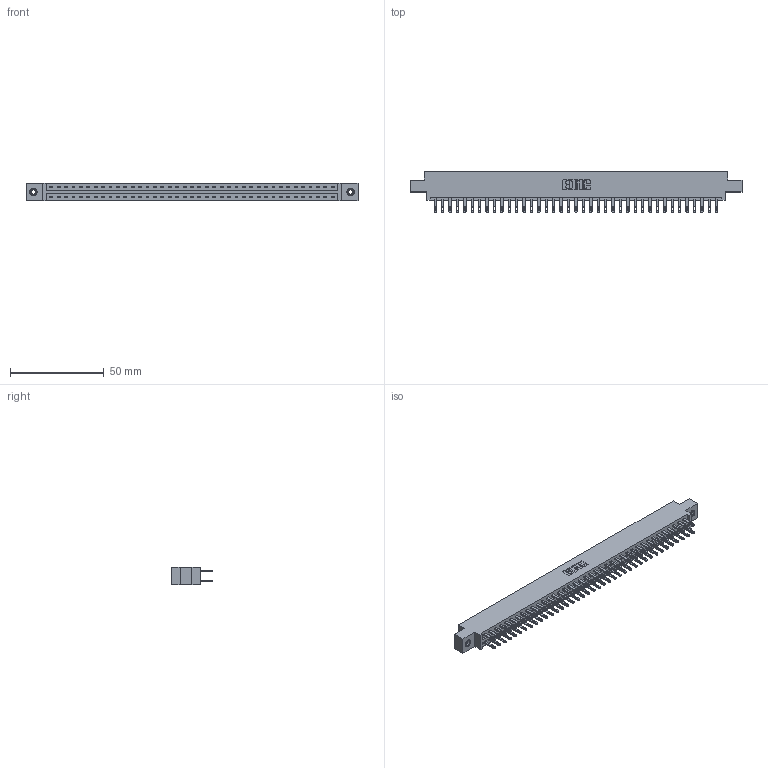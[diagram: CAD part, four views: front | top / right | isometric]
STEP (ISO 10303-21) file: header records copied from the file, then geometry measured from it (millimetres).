
FILE_DESCRIPTION (( 'STEP AP203' ), '1' );
FILE_NAME ('887-078-500-808.STEP', '2020-09-21T04:14:15', ( '' ), ( '' ), 'SwSTEP 2.0', 'SolidWorks 2020', '' );
FILE_SCHEMA (( 'CONFIG_CONTROL_DESIGN' ));
Length unit declared in the file: inch
Products named in the file (4): 345-292-001_345-293-100; 837 Part_0.170 Offset - 0.156 Dia-TI; 887-078-500-808; 345-250-001_345-250-003-102
Assembly tree (81 placements, depth 2):
  887-078-500-808
    837 Part_0.170 Offset - 0.156 Dia-TI
    345-292-001_345-293-100  x78
    345-250-001_345-250-003-102  x2
Bounding box: 177.55 x 21.85 x 9.4 mm (x, y, z)
Volume: 18785.6 mm3; surface area: 22205.3 mm2
Topology: 81 solids, 81 shells, 4078 faces, 12393 edges, 8254 vertices
Faces by surface type: plane 2602, cylinder 1460, cone 12, torus 4
Entity records: 31874 total; most frequent: CARTESIAN_POINT 5353, ORIENTED_EDGE 5282, DIRECTION 4591, EDGE_CURVE 2641, LINE 2489, VECTOR 2489, VERTEX_POINT 1756, AXIS2_PLACEMENT_3D 1051
